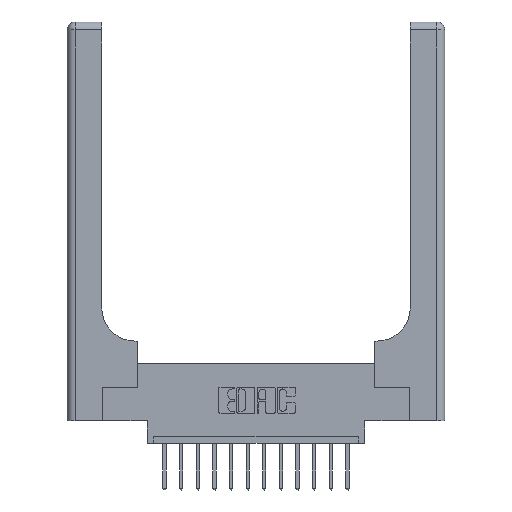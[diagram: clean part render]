
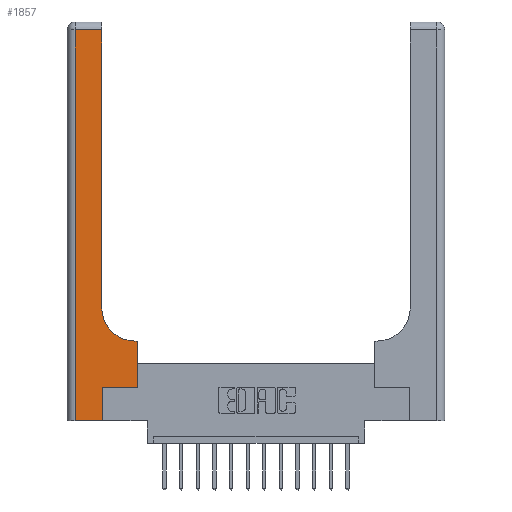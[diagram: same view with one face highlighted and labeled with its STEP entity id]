
A CAD part, top view. The second image highlights one B-rep face of the part: STEP entity #1857.
In plain terms, the highlighted planar face has unit normal (0, 0, 1).
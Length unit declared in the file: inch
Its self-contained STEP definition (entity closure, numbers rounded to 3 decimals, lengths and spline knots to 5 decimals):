
#227 = CARTESIAN_POINT ( 'NONE',  ( 0.528, 0.25, 0.37 ) ) ;
#654 = EDGE_CURVE ( 'NONE', #11323, #15575, #12855, .T. ) ;
#947 = DIRECTION ( 'NONE',  ( 1., 0., 0. ) ) ;
#953 = ORIENTED_EDGE ( 'NONE', *, *, #3570, .T. ) ;
#1013 = CARTESIAN_POINT ( 'NONE',  ( 0.265, 0., 0.37 ) ) ;
#1420 = DIRECTION ( 'NONE',  ( 1., 0., 0. ) ) ;
#1494 = EDGE_CURVE ( 'NONE', #15575, #16374, #3756, .T. ) ;
#1857 = ADVANCED_FACE ( 'NONE', ( #10210 ), #1972, .F. ) ;
#1972 = PLANE ( 'NONE',  #13790 ) ;
#2082 = LINE ( 'NONE', #1013, #5901 ) ;
#2085 = DIRECTION ( 'NONE',  ( 0., -1., 0. ) ) ;
#2664 = CARTESIAN_POINT ( 'NONE',  ( 0.26, 0.6, 0.37 ) ) ;
#2670 = CARTESIAN_POINT ( 'NONE',  ( 0.528, 0.6, 0.37 ) ) ;
#2916 = VECTOR ( 'NONE', #947, 39.37008 ) ;
#3213 = DIRECTION ( 'NONE',  ( -1., 0., 0. ) ) ;
#3214 = VERTEX_POINT ( 'NONE', #13645 ) ;
#3495 = CARTESIAN_POINT ( 'NONE',  ( 0.06, 3., 0.37 ) ) ;
#3570 = EDGE_CURVE ( 'NONE', #3214, #11323, #13624, .T. ) ;
#3623 = CARTESIAN_POINT ( 'NONE',  ( 0.528, 0.25, 0.37 ) ) ;
#3756 = LINE ( 'NONE', #9976, #2916 ) ;
#4506 = EDGE_CURVE ( 'NONE', #16374, #8141, #2082, .T. ) ;
#4620 = VERTEX_POINT ( 'NONE', #12790 ) ;
#4654 = ORIENTED_EDGE ( 'NONE', *, *, #14508, .T. ) ;
#5366 = VERTEX_POINT ( 'NONE', #2670 ) ;
#5555 = VERTEX_POINT ( 'NONE', #3623 ) ;
#5559 = VECTOR ( 'NONE', #11425, 39.37008 ) ;
#5691 = EDGE_CURVE ( 'NONE', #8141, #5555, #13794, .T. ) ;
#5794 = VECTOR ( 'NONE', #12124, 39.37008 ) ;
#5901 = VECTOR ( 'NONE', #8856, 39.37008 ) ;
#6099 = CARTESIAN_POINT ( 'NONE',  ( 0.06, 0., 0.37 ) ) ;
#6180 = EDGE_LOOP ( 'NONE', ( #16496, #953, #9929, #6845, #14141, #10245, #8812, #4654, #14483 ) ) ;
#6786 = LINE ( 'NONE', #12612, #5559 ) ;
#6845 = ORIENTED_EDGE ( 'NONE', *, *, #1494, .T. ) ;
#6999 = CARTESIAN_POINT ( 'NONE',  ( 0.06, 2.94, 0.37 ) ) ;
#7201 = CARTESIAN_POINT ( 'NONE',  ( 0.265, 0., 0.37 ) ) ;
#8141 = VERTEX_POINT ( 'NONE', #9588 ) ;
#8230 = VECTOR ( 'NONE', #2085, 39.37008 ) ;
#8232 = CARTESIAN_POINT ( 'NONE',  ( 0., 3., 0.37 ) ) ;
#8520 = LINE ( 'NONE', #2664, #11334 ) ;
#8812 = ORIENTED_EDGE ( 'NONE', *, *, #9970, .T. ) ;
#8856 = DIRECTION ( 'NONE',  ( 0., 1., 0. ) ) ;
#8947 = VECTOR ( 'NONE', #1420, 39.37008 ) ;
#9005 = DIRECTION ( 'NONE',  ( 1., 0., 0. ) ) ;
#9588 = CARTESIAN_POINT ( 'NONE',  ( 0.265, 0.25, 0.37 ) ) ;
#9929 = ORIENTED_EDGE ( 'NONE', *, *, #654, .T. ) ;
#9970 = EDGE_CURVE ( 'NONE', #5555, #5366, #12474, .T. ) ;
#9976 = CARTESIAN_POINT ( 'NONE',  ( 0., 0., 0.37 ) ) ;
#10171 = DIRECTION ( 'NONE',  ( 0., 0., -1. ) ) ;
#10210 = FACE_OUTER_BOUND ( 'NONE', #6180, .T. ) ;
#10245 = ORIENTED_EDGE ( 'NONE', *, *, #5691, .T. ) ;
#10629 = AXIS2_PLACEMENT_3D ( 'NONE', #12825, #10171, #9005 ) ;
#11158 = VERTEX_POINT ( 'NONE', #16344 ) ;
#11323 = VERTEX_POINT ( 'NONE', #6999 ) ;
#11334 = VECTOR ( 'NONE', #14355, 39.37008 ) ;
#11352 = CIRCLE ( 'NONE', #10629, 0.25 ) ;
#11425 = DIRECTION ( 'NONE',  ( 0., 1., 0. ) ) ;
#11597 = CARTESIAN_POINT ( 'NONE',  ( 0., 2.94, 0.37 ) ) ;
#11620 = EDGE_CURVE ( 'NONE', #4620, #11158, #11352, .T. ) ;
#11667 = DIRECTION ( 'NONE',  ( -1., 0., 0. ) ) ;
#12124 = DIRECTION ( 'NONE',  ( 0., 1., 0. ) ) ;
#12474 = LINE ( 'NONE', #227, #5794 ) ;
#12612 = CARTESIAN_POINT ( 'NONE',  ( 0.26, 3., 0.37 ) ) ;
#12790 = CARTESIAN_POINT ( 'NONE',  ( 0.51, 0.6, 0.37 ) ) ;
#12825 = CARTESIAN_POINT ( 'NONE',  ( 0.51, 0.85, 0.37 ) ) ;
#12855 = LINE ( 'NONE', #3495, #8230 ) ;
#12999 = VECTOR ( 'NONE', #11667, 39.37008 ) ;
#13012 = CARTESIAN_POINT ( 'NONE',  ( 0.265, 0.25, 0.37 ) ) ;
#13624 = LINE ( 'NONE', #11597, #12999 ) ;
#13645 = CARTESIAN_POINT ( 'NONE',  ( 0.26, 2.94, 0.37 ) ) ;
#13790 = AXIS2_PLACEMENT_3D ( 'NONE', #8232, #14730, #3213 ) ;
#13794 = LINE ( 'NONE', #13012, #8947 ) ;
#14141 = ORIENTED_EDGE ( 'NONE', *, *, #4506, .T. ) ;
#14355 = DIRECTION ( 'NONE',  ( -1., 0., 0. ) ) ;
#14483 = ORIENTED_EDGE ( 'NONE', *, *, #11620, .T. ) ;
#14508 = EDGE_CURVE ( 'NONE', #5366, #4620, #8520, .T. ) ;
#14730 = DIRECTION ( 'NONE',  ( 0., 0., -1. ) ) ;
#15575 = VERTEX_POINT ( 'NONE', #6099 ) ;
#16344 = CARTESIAN_POINT ( 'NONE',  ( 0.26, 0.85, 0.37 ) ) ;
#16374 = VERTEX_POINT ( 'NONE', #7201 ) ;
#16495 = EDGE_CURVE ( 'NONE', #11158, #3214, #6786, .T. ) ;
#16496 = ORIENTED_EDGE ( 'NONE', *, *, #16495, .T. ) ;
